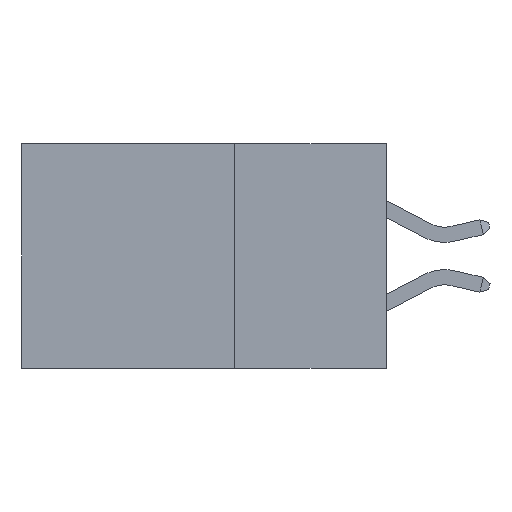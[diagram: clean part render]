
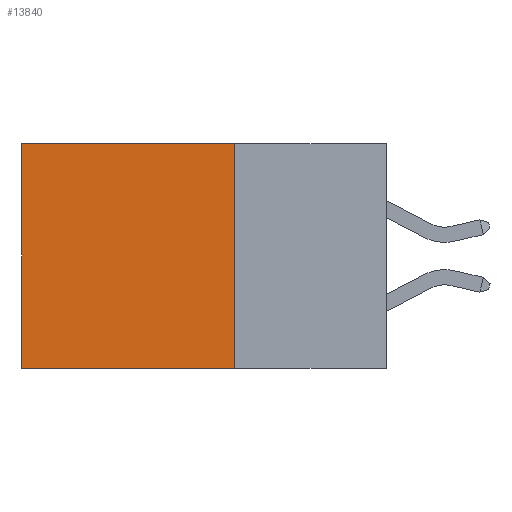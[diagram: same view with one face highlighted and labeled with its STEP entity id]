
A CAD part, left-side view. The second image highlights one B-rep face of the part: STEP entity #13840.
In plain terms, the highlighted planar face has unit normal (-1, 0, 0).
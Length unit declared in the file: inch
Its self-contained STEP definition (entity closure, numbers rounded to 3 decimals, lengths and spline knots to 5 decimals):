
#60 = ORIENTED_EDGE ( 'NONE', *, *, #12514, .F. ) ;
#728 = DIRECTION ( 'NONE',  ( 0., 1., 0. ) ) ;
#892 = VECTOR ( 'NONE', #15087, 39.37008 ) ;
#2452 = DIRECTION ( 'NONE',  ( 1., 0., 0. ) ) ;
#2509 = CARTESIAN_POINT ( 'NONE',  ( 0.298, 0.25, 0. ) ) ;
#2667 = CARTESIAN_POINT ( 'NONE',  ( 0.298, 0.25, 0. ) ) ;
#3204 = ORIENTED_EDGE ( 'NONE', *, *, #11072, .T. ) ;
#3294 = CARTESIAN_POINT ( 'NONE',  ( 0.298, 0.25, -0.37 ) ) ;
#3322 = VERTEX_POINT ( 'NONE', #2667 ) ;
#3508 = ORIENTED_EDGE ( 'NONE', *, *, #8761, .F. ) ;
#3841 = LINE ( 'NONE', #14810, #10354 ) ;
#4440 = CARTESIAN_POINT ( 'NONE',  ( 0.298, 0.6, 0. ) ) ;
#5291 = EDGE_CURVE ( 'NONE', #3322, #16800, #5878, .T. ) ;
#5878 = LINE ( 'NONE', #18651, #14714 ) ;
#7505 = VERTEX_POINT ( 'NONE', #18169 ) ;
#7788 = CARTESIAN_POINT ( 'NONE',  ( 0.298, 0.6, 0. ) ) ;
#8402 = DIRECTION ( 'NONE',  ( 0., 0., -1. ) ) ;
#8761 = EDGE_CURVE ( 'NONE', #7505, #17506, #17620, .T. ) ;
#10354 = VECTOR ( 'NONE', #14749, 39.37008 ) ;
#11072 = EDGE_CURVE ( 'NONE', #16800, #17506, #17806, .T. ) ;
#12496 = CARTESIAN_POINT ( 'NONE',  ( 0.298, 0.6, -0.37 ) ) ;
#12514 = EDGE_CURVE ( 'NONE', #3322, #7505, #3841, .T. ) ;
#13018 = PLANE ( 'NONE',  #15375 ) ;
#13840 = ADVANCED_FACE ( 'NONE', ( #18431 ), #13018, .F. ) ;
#14650 = EDGE_LOOP ( 'NONE', ( #3204, #3508, #60, #15732 ) ) ;
#14714 = VECTOR ( 'NONE', #728, 39.37008 ) ;
#14749 = DIRECTION ( 'NONE',  ( 0., 0., -1. ) ) ;
#14810 = CARTESIAN_POINT ( 'NONE',  ( 0.298, 0.25, 0. ) ) ;
#15087 = DIRECTION ( 'NONE',  ( 0., 1., 0. ) ) ;
#15375 = AXIS2_PLACEMENT_3D ( 'NONE', #2509, #2452, #8402 ) ;
#15732 = ORIENTED_EDGE ( 'NONE', *, *, #5291, .T. ) ;
#15926 = VECTOR ( 'NONE', #16388, 39.37008 ) ;
#16388 = DIRECTION ( 'NONE',  ( 0., 0., -1. ) ) ;
#16800 = VERTEX_POINT ( 'NONE', #7788 ) ;
#17506 = VERTEX_POINT ( 'NONE', #12496 ) ;
#17620 = LINE ( 'NONE', #3294, #892 ) ;
#17806 = LINE ( 'NONE', #4440, #15926 ) ;
#18169 = CARTESIAN_POINT ( 'NONE',  ( 0.298, 0.25, -0.37 ) ) ;
#18431 = FACE_OUTER_BOUND ( 'NONE', #14650, .T. ) ;
#18651 = CARTESIAN_POINT ( 'NONE',  ( 0.298, 0.25, 0. ) ) ;
